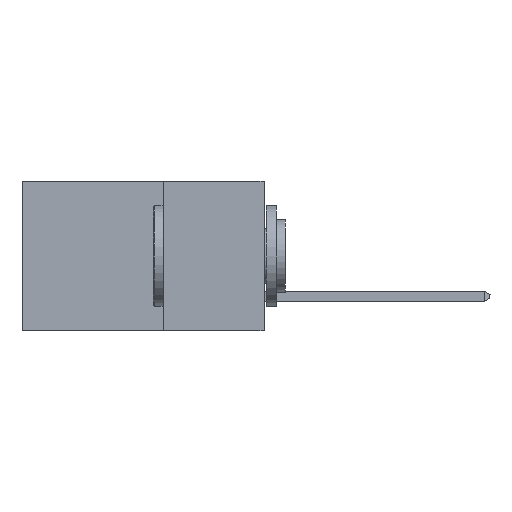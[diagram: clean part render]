
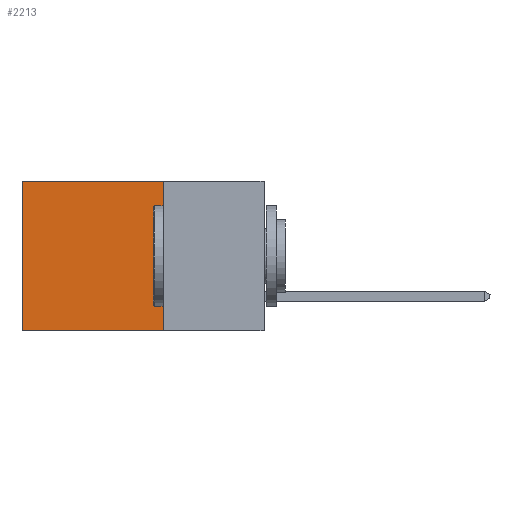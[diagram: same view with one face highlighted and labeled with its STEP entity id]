
A CAD part, left-side view. The second image highlights one B-rep face of the part: STEP entity #2213.
In plain terms, the highlighted planar face has unit normal (-1, 0, 0).
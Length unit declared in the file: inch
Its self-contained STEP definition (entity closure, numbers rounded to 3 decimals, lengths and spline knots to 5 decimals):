
#41 = ORIENTED_EDGE ( 'NONE', *, *, #2558, .T. ) ;
#411 = CARTESIAN_POINT ( 'NONE',  ( 0.2615, 0.25, -0.37 ) ) ;
#658 = EDGE_CURVE ( 'NONE', #3005, #1491, #9374, .T. ) ;
#677 = CARTESIAN_POINT ( 'NONE',  ( 0.2615, 0.6, -0.37 ) ) ;
#797 = CARTESIAN_POINT ( 'NONE',  ( 0.2615, 0.25, -0.37 ) ) ;
#1491 = VERTEX_POINT ( 'NONE', #6570 ) ;
#1632 = LINE ( 'NONE', #677, #6582 ) ;
#2096 = CARTESIAN_POINT ( 'NONE',  ( 0.2615, 0.25, 0. ) ) ;
#2142 = LINE ( 'NONE', #8383, #5108 ) ;
#2186 = CARTESIAN_POINT ( 'NONE',  ( 0.2615, 0.25, -0.37 ) ) ;
#2213 = ADVANCED_FACE ( 'NONE', ( #4084 ), #5030, .F. ) ;
#2558 = EDGE_CURVE ( 'NONE', #9505, #1491, #1632, .T. ) ;
#2573 = LINE ( 'NONE', #411, #7220 ) ;
#3005 = VERTEX_POINT ( 'NONE', #797 ) ;
#3914 = VECTOR ( 'NONE', #8604, 39.37008 ) ;
#4084 = FACE_OUTER_BOUND ( 'NONE', #4377, .T. ) ;
#4377 = EDGE_LOOP ( 'NONE', ( #41, #9042, #11693, #12278 ) ) ;
#5030 = PLANE ( 'NONE',  #11551 ) ;
#5108 = VECTOR ( 'NONE', #5193, 39.37008 ) ;
#5193 = DIRECTION ( 'NONE',  ( 0., 1., 0. ) ) ;
#5629 = DIRECTION ( 'NONE',  ( 0., 0., -1. ) ) ;
#6570 = CARTESIAN_POINT ( 'NONE',  ( 0.2615, 0.6, -0.37 ) ) ;
#6582 = VECTOR ( 'NONE', #6715, 39.37008 ) ;
#6715 = DIRECTION ( 'NONE',  ( 0., 0., -1. ) ) ;
#7220 = VECTOR ( 'NONE', #5629, 39.37008 ) ;
#8383 = CARTESIAN_POINT ( 'NONE',  ( 0.2615, 0.25, 0. ) ) ;
#8604 = DIRECTION ( 'NONE',  ( 0., 1., 0. ) ) ;
#9042 = ORIENTED_EDGE ( 'NONE', *, *, #658, .F. ) ;
#9157 = DIRECTION ( 'NONE',  ( 1., 0., 0. ) ) ;
#9374 = LINE ( 'NONE', #2186, #3914 ) ;
#9505 = VERTEX_POINT ( 'NONE', #12821 ) ;
#11432 = EDGE_CURVE ( 'NONE', #12972, #3005, #2573, .T. ) ;
#11439 = DIRECTION ( 'NONE',  ( 0., 0., -1. ) ) ;
#11551 = AXIS2_PLACEMENT_3D ( 'NONE', #12317, #9157, #11439 ) ;
#11693 = ORIENTED_EDGE ( 'NONE', *, *, #11432, .F. ) ;
#12278 = ORIENTED_EDGE ( 'NONE', *, *, #13329, .T. ) ;
#12317 = CARTESIAN_POINT ( 'NONE',  ( 0.2615, 0.25, -0.37 ) ) ;
#12821 = CARTESIAN_POINT ( 'NONE',  ( 0.2615, 0.6, 0. ) ) ;
#12972 = VERTEX_POINT ( 'NONE', #2096 ) ;
#13329 = EDGE_CURVE ( 'NONE', #12972, #9505, #2142, .T. ) ;
